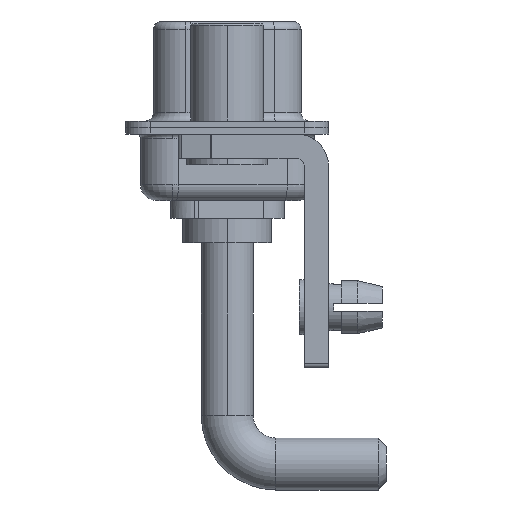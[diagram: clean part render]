
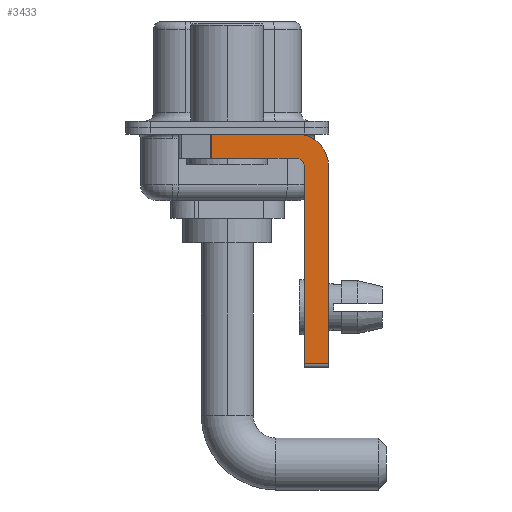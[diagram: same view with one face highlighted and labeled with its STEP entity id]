
A CAD part, left-side view. The second image highlights one B-rep face of the part: STEP entity #3433.
In plain terms, the highlighted planar face has unit normal (-1, 0, 0).
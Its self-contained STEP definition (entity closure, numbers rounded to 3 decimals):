
#160 = DIRECTION ( 'NONE',  ( 0., 0., -1. ) ) ;
#430 = ORIENTED_EDGE ( 'NONE', *, *, #18852, .F. ) ;
#505 = CARTESIAN_POINT ( 'NONE',  ( -2.9, -4.25, -14.55 ) ) ;
#557 = DIRECTION ( 'NONE',  ( 0., 1., 0. ) ) ;
#1275 = CARTESIAN_POINT ( 'NONE',  ( -2.9, -6.25, -2.4 ) ) ;
#1455 = VERTEX_POINT ( 'NONE', #6046 ) ;
#1503 = CARTESIAN_POINT ( 'NONE',  ( -2.9, -4.75, -14.55 ) ) ;
#1803 = AXIS2_PLACEMENT_3D ( 'NONE', #14081, #15707, #160 ) ;
#1810 = DIRECTION ( 'NONE',  ( 0., 0., -1. ) ) ;
#2013 = LINE ( 'NONE', #11341, #19667 ) ;
#2040 = DIRECTION ( 'NONE',  ( 0., -1., 0. ) ) ;
#2310 = VERTEX_POINT ( 'NONE', #1503 ) ;
#2462 = EDGE_CURVE ( 'NONE', #2310, #17042, #2013, .T. ) ;
#3073 = ORIENTED_EDGE ( 'NONE', *, *, #16115, .T. ) ;
#3352 = DIRECTION ( 'NONE',  ( 0., -1., 0. ) ) ;
#3433 = ADVANCED_FACE ( 'NONE', ( #19291 ), #8055, .F. ) ;
#3735 = EDGE_CURVE ( 'NONE', #15577, #4527, #10802, .T. ) ;
#3781 = ORIENTED_EDGE ( 'NONE', *, *, #3868, .F. ) ;
#3868 = EDGE_CURVE ( 'NONE', #8810, #6803, #9671, .T. ) ;
#4130 = ORIENTED_EDGE ( 'NONE', *, *, #9127, .T. ) ;
#4389 = VECTOR ( 'NONE', #3352, 1000. ) ;
#4527 = VERTEX_POINT ( 'NONE', #14650 ) ;
#4889 = VECTOR ( 'NONE', #557, 1000. ) ;
#5691 = CARTESIAN_POINT ( 'NONE',  ( -2.9, 0.978, -1.9 ) ) ;
#6046 = CARTESIAN_POINT ( 'NONE',  ( -2.9, 0.978, -0.4 ) ) ;
#6166 = DIRECTION ( 'NONE',  ( -1., 0., 0. ) ) ;
#6803 = VERTEX_POINT ( 'NONE', #19065 ) ;
#6842 = LINE ( 'NONE', #505, #19607 ) ;
#7457 = VECTOR ( 'NONE', #15596, 1000. ) ;
#7633 = DIRECTION ( 'NONE',  ( 0., 0., -1. ) ) ;
#7871 = CARTESIAN_POINT ( 'NONE',  ( -2.9, -4.75, -2.4 ) ) ;
#8055 = PLANE ( 'NONE',  #17907 ) ;
#8810 = VERTEX_POINT ( 'NONE', #15245 ) ;
#9127 = EDGE_CURVE ( 'NONE', #2310, #4527, #6842, .T. ) ;
#9671 = LINE ( 'NONE', #18973, #4889 ) ;
#9892 = DIRECTION ( 'NONE',  ( 1., 0., 0. ) ) ;
#10132 = CARTESIAN_POINT ( 'NONE',  ( -2.9, -6.25, -2.4 ) ) ;
#10529 = CARTESIAN_POINT ( 'NONE',  ( -2.9, -4.25, -0.4 ) ) ;
#10802 = LINE ( 'NONE', #1275, #7457 ) ;
#10842 = VERTEX_POINT ( 'NONE', #10529 ) ;
#11236 = DIRECTION ( 'NONE',  ( 0., 0., 1. ) ) ;
#11341 = CARTESIAN_POINT ( 'NONE',  ( -2.9, -4.75, -14.8 ) ) ;
#12065 = ORIENTED_EDGE ( 'NONE', *, *, #3735, .F. ) ;
#12092 = EDGE_LOOP ( 'NONE', ( #430, #3073, #3781, #13868, #19757, #4130, #12065, #15183 ) ) ;
#13852 = EDGE_CURVE ( 'NONE', #17042, #8810, #15451, .T. ) ;
#13868 = ORIENTED_EDGE ( 'NONE', *, *, #13852, .F. ) ;
#14081 = CARTESIAN_POINT ( 'NONE',  ( -2.9, -4.25, -2.4 ) ) ;
#14650 = CARTESIAN_POINT ( 'NONE',  ( -2.9, -6.25, -14.55 ) ) ;
#14883 = VECTOR ( 'NONE', #7633, 1000. ) ;
#15183 = ORIENTED_EDGE ( 'NONE', *, *, #16347, .F. ) ;
#15245 = CARTESIAN_POINT ( 'NONE',  ( -2.9, -4.25, -1.9 ) ) ;
#15451 = CIRCLE ( 'NONE', #16771, 0.5 ) ;
#15577 = VERTEX_POINT ( 'NONE', #10132 ) ;
#15596 = DIRECTION ( 'NONE',  ( 0., 0., -1. ) ) ;
#15707 = DIRECTION ( 'NONE',  ( 1., 0., 0. ) ) ;
#16115 = EDGE_CURVE ( 'NONE', #1455, #6803, #18484, .T. ) ;
#16347 = EDGE_CURVE ( 'NONE', #10842, #15577, #19435, .T. ) ;
#16771 = AXIS2_PLACEMENT_3D ( 'NONE', #18949, #6166, #17225 ) ;
#17042 = VERTEX_POINT ( 'NONE', #7871 ) ;
#17225 = DIRECTION ( 'NONE',  ( 0., 0., 1. ) ) ;
#17276 = CARTESIAN_POINT ( 'NONE',  ( -2.9, 3., -0.4 ) ) ;
#17373 = LINE ( 'NONE', #17276, #4389 ) ;
#17665 = CARTESIAN_POINT ( 'NONE',  ( -2.9, -4.25, -2.4 ) ) ;
#17907 = AXIS2_PLACEMENT_3D ( 'NONE', #17665, #9892, #1810 ) ;
#18484 = LINE ( 'NONE', #5691, #14883 ) ;
#18852 = EDGE_CURVE ( 'NONE', #1455, #10842, #17373, .T. ) ;
#18949 = CARTESIAN_POINT ( 'NONE',  ( -2.9, -4.25, -2.4 ) ) ;
#18973 = CARTESIAN_POINT ( 'NONE',  ( -2.9, -4.25, -1.9 ) ) ;
#19065 = CARTESIAN_POINT ( 'NONE',  ( -2.9, 0.978, -1.9 ) ) ;
#19291 = FACE_OUTER_BOUND ( 'NONE', #12092, .T. ) ;
#19435 = CIRCLE ( 'NONE', #1803, 2. ) ;
#19607 = VECTOR ( 'NONE', #2040, 1000. ) ;
#19667 = VECTOR ( 'NONE', #11236, 1000. ) ;
#19757 = ORIENTED_EDGE ( 'NONE', *, *, #2462, .F. ) ;
